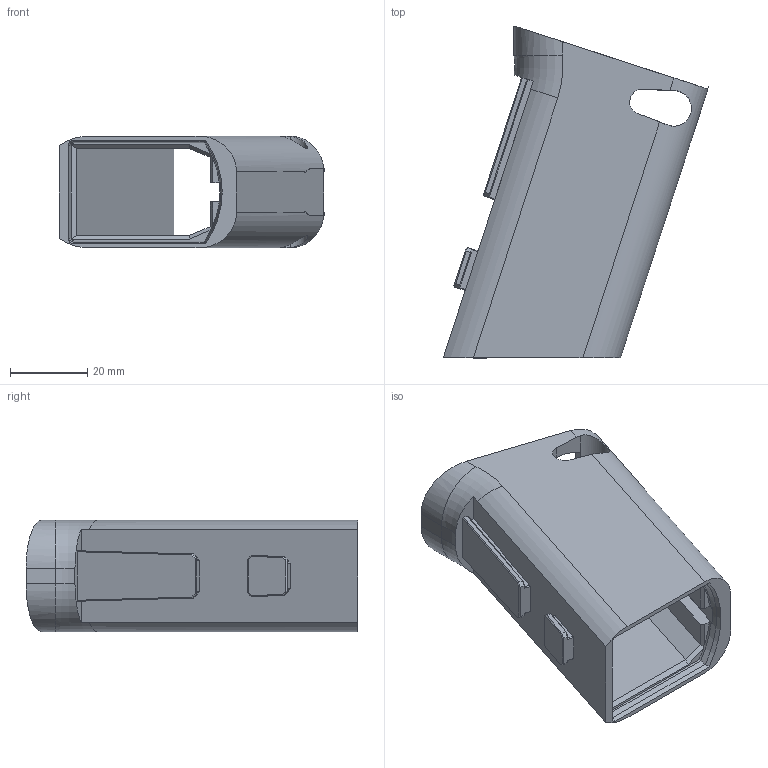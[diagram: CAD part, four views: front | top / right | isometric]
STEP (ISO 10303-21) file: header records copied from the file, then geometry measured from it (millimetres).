
FILE_DESCRIPTION(/* description */ (''),/* implementation_level */ '2;1');
FILE_NAME(/* name */ 'FNS-940_Magwell_1 v1.step',/* time_stamp */ '2021-06-04T19:32:38-07:00',/* author */ (''),/* organization */ (''),/* preprocessor_version */ 'ST-DEVELOPER v18.1',/* originating_system */ 'Autodesk Translation Framework v10.9.0.1377',/* authorisation */ '');
FILE_SCHEMA (('AUTOMOTIVE_DESIGN { 1 0 10303 214 3 1 1 }'));
Length unit declared in the file: millimetre
Products named in the file (5): FNS-940_Magwell_1; Main Frame; Compact Size Grip; Standard Size Grip; Standard Size Grip (Stopgap)
Assembly tree (4 placements, depth 2):
  FNS-940_Magwell_1
    Main Frame
    Compact Size Grip
    Standard Size Grip
    Standard Size Grip (Stopgap)
Bounding box: 68.88 x 86.17 x 29 mm (x, y, z)
Volume: 38200.2 mm3; surface area: 21822.7 mm2
Topology: 1 solids, 1 shells, 150 faces, 423 edges, 272 vertices
Faces by surface type: plane 120, cylinder 18, torus 6, cone 4, bspline 2
Entity records: 5210 total; most frequent: CARTESIAN_POINT 1177, ORIENTED_EDGE 846, DIRECTION 784, EDGE_CURVE 423, LINE 328, VECTOR 328, VERTEX_POINT 272, AXIS2_PLACEMENT_3D 228
